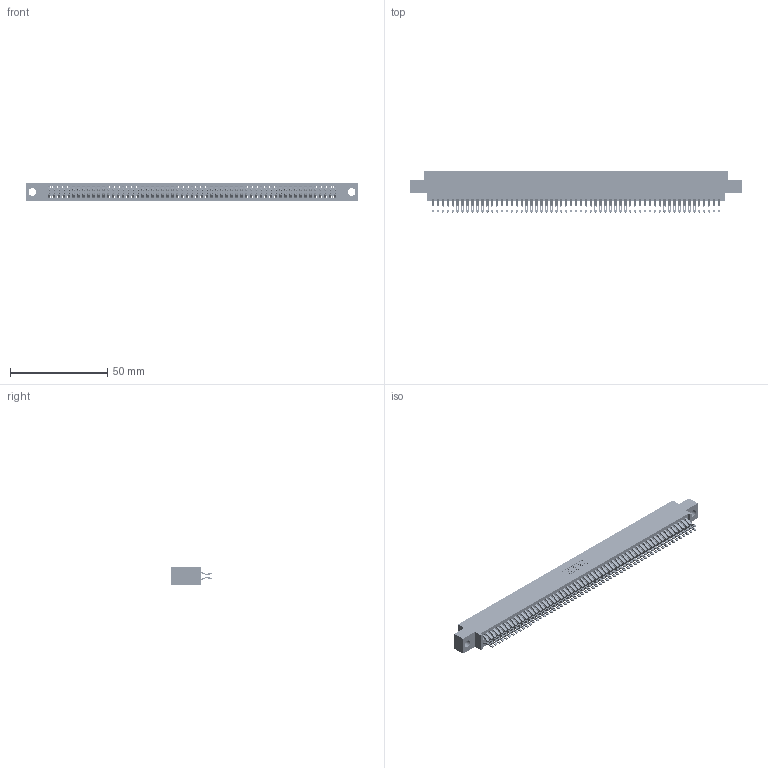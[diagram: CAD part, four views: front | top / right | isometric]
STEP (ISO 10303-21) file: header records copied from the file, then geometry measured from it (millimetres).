
FILE_DESCRIPTION (( 'STEP AP203' ), '1' );
FILE_NAME ('395-118-555-804.STEP', '2018-12-02T09:44:53', ( '' ), ( '' ), 'SwSTEP 2.0', 'SolidWorks 2016', '' );
FILE_SCHEMA (( 'CONFIG_CONTROL_DESIGN' ));
Length unit declared in the file: inch
Products named in the file (3): 395-118-555-804; 345 Part_0.170 Offset - 0.156 Dia-TH; 345-292-001_555 Tail
Assembly tree (119 placements, depth 2):
  395-118-555-804
    345 Part_0.170 Offset - 0.156 Dia-TH
    345-292-001_555 Tail  x118
Bounding box: 171.07 x 21.13 x 9.4 mm (x, y, z)
Volume: 16916.6 mm3; surface area: 26484 mm2
Topology: 119 solids, 119 shells, 6738 faces, 21239 edges, 14158 vertices
Faces by surface type: plane 3742, cylinder 2996
Entity records: 44465 total; most frequent: CARTESIAN_POINT 7474, ORIENTED_EDGE 7378, DIRECTION 6537, EDGE_CURVE 3689, LINE 3301, VECTOR 3301, VERTEX_POINT 2458, AXIS2_PLACEMENT_3D 1618
